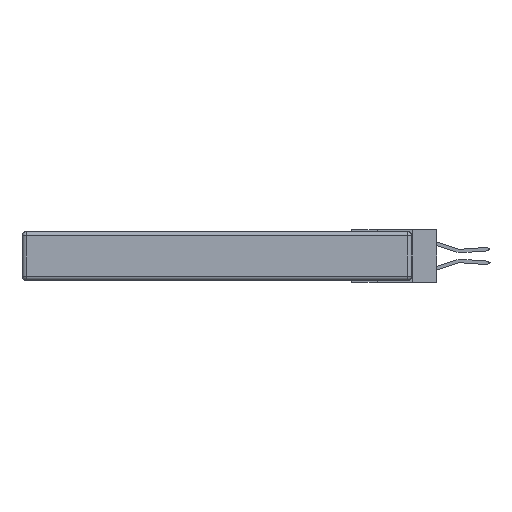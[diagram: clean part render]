
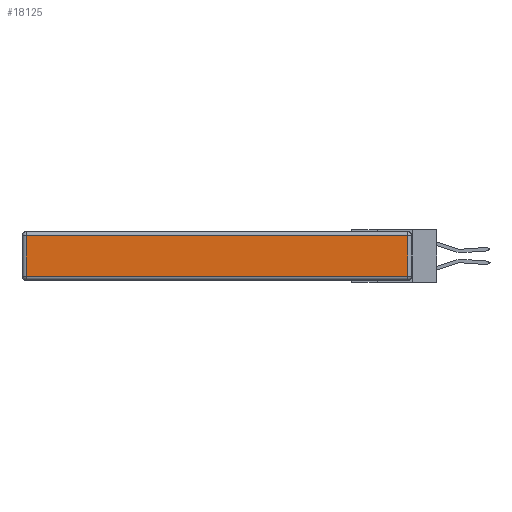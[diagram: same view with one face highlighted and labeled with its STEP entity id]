
A CAD part, left-side view. The second image highlights one B-rep face of the part: STEP entity #18125.
In plain terms, the highlighted planar face has unit normal (-1, 0, 0).
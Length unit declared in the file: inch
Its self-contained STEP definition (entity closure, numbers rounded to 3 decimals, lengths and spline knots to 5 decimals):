
#2669 = LINE ( 'NONE', #9398, #2901 ) ;
#2901 = VECTOR ( 'NONE', #6746, 39.37008 ) ;
#2956 = ORIENTED_EDGE ( 'NONE', *, *, #12372, .T. ) ;
#3408 = EDGE_CURVE ( 'NONE', #13857, #12751, #13536, .T. ) ;
#3466 = FACE_OUTER_BOUND ( 'NONE', #4943, .T. ) ;
#4264 = VECTOR ( 'NONE', #15145, 39.37008 ) ;
#4737 = LINE ( 'NONE', #16630, #4264 ) ;
#4943 = EDGE_LOOP ( 'NONE', ( #2956, #15224, #6302, #10063 ) ) ;
#5550 = CARTESIAN_POINT ( 'NONE',  ( 0., 0.03, -0.343 ) ) ;
#5985 = CARTESIAN_POINT ( 'NONE',  ( 0., 0.03, -0.313 ) ) ;
#6260 = DIRECTION ( 'NONE',  ( -1., 0., 0. ) ) ;
#6302 = ORIENTED_EDGE ( 'NONE', *, *, #11461, .T. ) ;
#6746 = DIRECTION ( 'NONE',  ( 0., -1., 0. ) ) ;
#7460 = VECTOR ( 'NONE', #15377, 39.37008 ) ;
#7519 = LINE ( 'NONE', #13223, #7738 ) ;
#7738 = VECTOR ( 'NONE', #8393, 39.37008 ) ;
#7985 = EDGE_CURVE ( 'NONE', #15983, #19834, #7519, .T. ) ;
#8393 = DIRECTION ( 'NONE',  ( 0., 0., -1. ) ) ;
#9114 = DIRECTION ( 'NONE',  ( 0., 0., 1. ) ) ;
#9398 = CARTESIAN_POINT ( 'NONE',  ( 0., 0., -0.313 ) ) ;
#10063 = ORIENTED_EDGE ( 'NONE', *, *, #7985, .T. ) ;
#10736 = CARTESIAN_POINT ( 'NONE',  ( 0., 0., -0.343 ) ) ;
#11461 = EDGE_CURVE ( 'NONE', #12751, #15983, #4737, .T. ) ;
#12372 = EDGE_CURVE ( 'NONE', #19834, #13857, #2669, .T. ) ;
#12411 = CARTESIAN_POINT ( 'NONE',  ( 0., 2.72, -0.313 ) ) ;
#12751 = VERTEX_POINT ( 'NONE', #15141 ) ;
#13223 = CARTESIAN_POINT ( 'NONE',  ( 0., 2.72, -0.343 ) ) ;
#13536 = LINE ( 'NONE', #5550, #7460 ) ;
#13857 = VERTEX_POINT ( 'NONE', #5985 ) ;
#15141 = CARTESIAN_POINT ( 'NONE',  ( 0., 0.03, -0.03 ) ) ;
#15145 = DIRECTION ( 'NONE',  ( 0., 1., 0. ) ) ;
#15224 = ORIENTED_EDGE ( 'NONE', *, *, #3408, .T. ) ;
#15262 = AXIS2_PLACEMENT_3D ( 'NONE', #10736, #6260, #9114 ) ;
#15377 = DIRECTION ( 'NONE',  ( 0., 0., 1. ) ) ;
#15983 = VERTEX_POINT ( 'NONE', #18454 ) ;
#16630 = CARTESIAN_POINT ( 'NONE',  ( 0., 2.75, -0.03 ) ) ;
#16968 = PLANE ( 'NONE',  #15262 ) ;
#18125 = ADVANCED_FACE ( 'NONE', ( #3466 ), #16968, .T. ) ;
#18454 = CARTESIAN_POINT ( 'NONE',  ( 0., 2.72, -0.03 ) ) ;
#19834 = VERTEX_POINT ( 'NONE', #12411 ) ;
